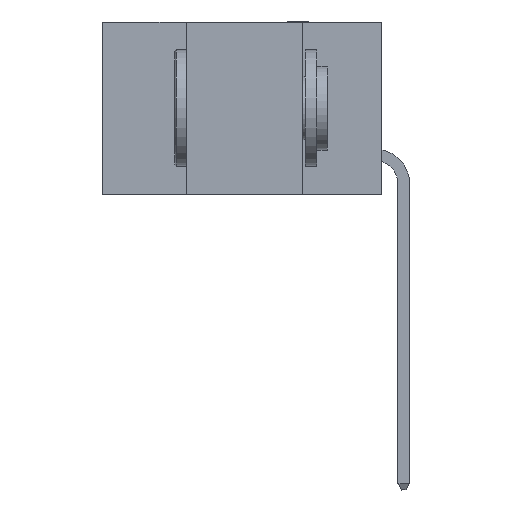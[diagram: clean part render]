
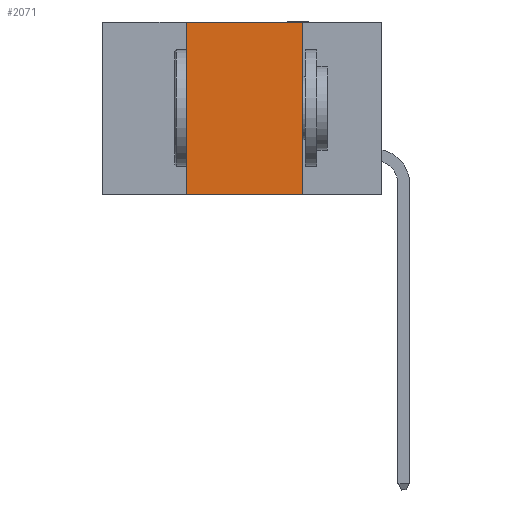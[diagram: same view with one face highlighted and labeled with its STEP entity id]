
A CAD part, left-side view. The second image highlights one B-rep face of the part: STEP entity #2071.
In plain terms, the highlighted planar face has unit normal (-1, 0, 0).
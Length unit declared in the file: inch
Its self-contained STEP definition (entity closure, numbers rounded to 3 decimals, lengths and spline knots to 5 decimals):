
#902 = LINE ( 'NONE', #28427, #18241 ) ;
#2071 = ADVANCED_FACE ( 'NONE', ( #4837 ), #27103, .F. ) ;
#2536 = CARTESIAN_POINT ( 'NONE',  ( 0., 0.42, 0. ) ) ;
#2697 = CARTESIAN_POINT ( 'NONE',  ( 0., 0.42, 0. ) ) ;
#3015 = EDGE_CURVE ( 'NONE', #32464, #7208, #902, .T. ) ;
#3498 = CARTESIAN_POINT ( 'NONE',  ( 0., 0.6, 0. ) ) ;
#4837 = FACE_OUTER_BOUND ( 'NONE', #12110, .T. ) ;
#5080 = VERTEX_POINT ( 'NONE', #17284 ) ;
#7208 = VERTEX_POINT ( 'NONE', #28316 ) ;
#7737 = DIRECTION ( 'NONE',  ( 0., 0., -1. ) ) ;
#8536 = DIRECTION ( 'NONE',  ( 0., 0., -1. ) ) ;
#10042 = VECTOR ( 'NONE', #39023, 39.37008 ) ;
#12110 = EDGE_LOOP ( 'NONE', ( #29830, #14151, #29820, #28973 ) ) ;
#13034 = DIRECTION ( 'NONE',  ( 0., -1., 0. ) ) ;
#14151 = ORIENTED_EDGE ( 'NONE', *, *, #29536, .F. ) ;
#14183 = CARTESIAN_POINT ( 'NONE',  ( 0., 0.17, 0. ) ) ;
#14722 = CARTESIAN_POINT ( 'NONE',  ( 0., 0.6, 0. ) ) ;
#15151 = CARTESIAN_POINT ( 'NONE',  ( 0., 0.6, -0.37 ) ) ;
#17284 = CARTESIAN_POINT ( 'NONE',  ( 0., 0.42, -0.37 ) ) ;
#18241 = VECTOR ( 'NONE', #7737, 39.37008 ) ;
#21687 = EDGE_CURVE ( 'NONE', #5080, #38525, #26397, .T. ) ;
#23442 = VECTOR ( 'NONE', #13034, 39.37008 ) ;
#23576 = AXIS2_PLACEMENT_3D ( 'NONE', #14722, #30300, #8536 ) ;
#25628 = VECTOR ( 'NONE', #36255, 39.37008 ) ;
#25992 = EDGE_CURVE ( 'NONE', #5080, #7208, #27065, .T. ) ;
#26328 = LINE ( 'NONE', #3498, #23442 ) ;
#26397 = LINE ( 'NONE', #2536, #10042 ) ;
#27065 = LINE ( 'NONE', #15151, #25628 ) ;
#27103 = PLANE ( 'NONE',  #23576 ) ;
#28316 = CARTESIAN_POINT ( 'NONE',  ( 0., 0.17, -0.37 ) ) ;
#28427 = CARTESIAN_POINT ( 'NONE',  ( 0., 0.17, 0. ) ) ;
#28973 = ORIENTED_EDGE ( 'NONE', *, *, #25992, .T. ) ;
#29536 = EDGE_CURVE ( 'NONE', #38525, #32464, #26328, .T. ) ;
#29820 = ORIENTED_EDGE ( 'NONE', *, *, #21687, .F. ) ;
#29830 = ORIENTED_EDGE ( 'NONE', *, *, #3015, .F. ) ;
#30300 = DIRECTION ( 'NONE',  ( 1., 0., 0. ) ) ;
#32464 = VERTEX_POINT ( 'NONE', #14183 ) ;
#36255 = DIRECTION ( 'NONE',  ( 0., -1., 0. ) ) ;
#38525 = VERTEX_POINT ( 'NONE', #2697 ) ;
#39023 = DIRECTION ( 'NONE',  ( 0., 0., 1. ) ) ;
